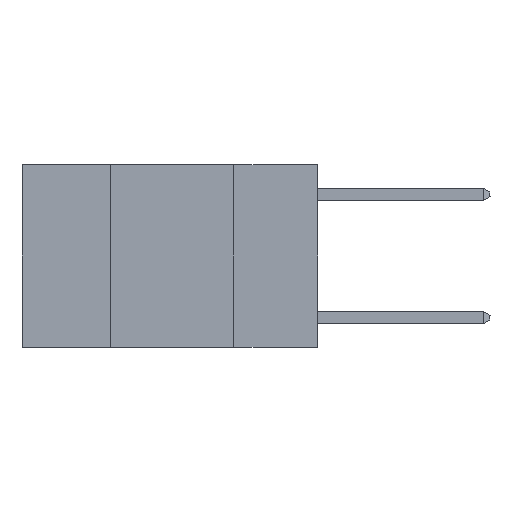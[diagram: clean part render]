
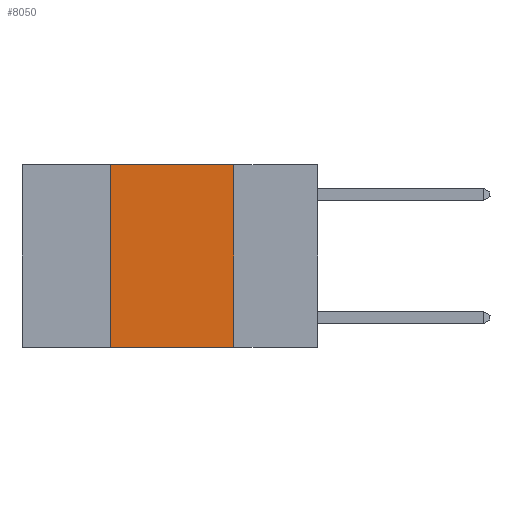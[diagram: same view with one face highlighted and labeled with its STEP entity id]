
A CAD part, left-side view. The second image highlights one B-rep face of the part: STEP entity #8050.
In plain terms, the highlighted planar face has unit normal (-1, 0, 0).
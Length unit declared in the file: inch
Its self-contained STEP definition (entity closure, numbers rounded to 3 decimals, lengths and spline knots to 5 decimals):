
#43 = AXIS2_PLACEMENT_3D ( 'NONE', #1854, #23886, #24026 ) ;
#94 = VECTOR ( 'NONE', #15990, 39.37008 ) ;
#1108 = EDGE_CURVE ( 'NONE', #13047, #16298, #21081, .T. ) ;
#1854 = CARTESIAN_POINT ( 'NONE',  ( 0., 0.6, 0. ) ) ;
#1896 = ORIENTED_EDGE ( 'NONE', *, *, #28391, .F. ) ;
#2667 = LINE ( 'NONE', #18173, #94 ) ;
#3849 = EDGE_CURVE ( 'NONE', #11766, #23685, #21653, .T. ) ;
#4004 = CARTESIAN_POINT ( 'NONE',  ( 0., 0.17, 0. ) ) ;
#4417 = VECTOR ( 'NONE', #8934, 39.37008 ) ;
#6445 = CARTESIAN_POINT ( 'NONE',  ( 0., 0.17, -0.37 ) ) ;
#7038 = VECTOR ( 'NONE', #18765, 39.37008 ) ;
#7938 = CARTESIAN_POINT ( 'NONE',  ( 0., 0.42, 0. ) ) ;
#8050 = ADVANCED_FACE ( 'NONE', ( #15036 ), #17356, .F. ) ;
#8934 = DIRECTION ( 'NONE',  ( 0., -1., 0. ) ) ;
#8973 = ORIENTED_EDGE ( 'NONE', *, *, #3849, .F. ) ;
#10432 = ORIENTED_EDGE ( 'NONE', *, *, #25284, .T. ) ;
#11766 = VERTEX_POINT ( 'NONE', #24717 ) ;
#13047 = VERTEX_POINT ( 'NONE', #16086 ) ;
#14161 = CARTESIAN_POINT ( 'NONE',  ( 0., 0.42, 0. ) ) ;
#15036 = FACE_OUTER_BOUND ( 'NONE', #17390, .T. ) ;
#15990 = DIRECTION ( 'NONE',  ( 0., -1., 0. ) ) ;
#16086 = CARTESIAN_POINT ( 'NONE',  ( 0., 0.42, -0.37 ) ) ;
#16298 = VERTEX_POINT ( 'NONE', #14161 ) ;
#16890 = LINE ( 'NONE', #26885, #4417 ) ;
#17356 = PLANE ( 'NONE',  #43 ) ;
#17390 = EDGE_LOOP ( 'NONE', ( #8973, #1896, #19580, #10432 ) ) ;
#18173 = CARTESIAN_POINT ( 'NONE',  ( 0., 0.6, -0.37 ) ) ;
#18765 = DIRECTION ( 'NONE',  ( 0., 0., 1. ) ) ;
#18779 = VECTOR ( 'NONE', #26297, 39.37008 ) ;
#19580 = ORIENTED_EDGE ( 'NONE', *, *, #1108, .F. ) ;
#21081 = LINE ( 'NONE', #7938, #7038 ) ;
#21653 = LINE ( 'NONE', #4004, #18779 ) ;
#23685 = VERTEX_POINT ( 'NONE', #6445 ) ;
#23886 = DIRECTION ( 'NONE',  ( 1., 0., 0. ) ) ;
#24026 = DIRECTION ( 'NONE',  ( 0., 0., -1. ) ) ;
#24717 = CARTESIAN_POINT ( 'NONE',  ( 0., 0.17, 0. ) ) ;
#25284 = EDGE_CURVE ( 'NONE', #13047, #23685, #2667, .T. ) ;
#26297 = DIRECTION ( 'NONE',  ( 0., 0., -1. ) ) ;
#26885 = CARTESIAN_POINT ( 'NONE',  ( 0., 0.6, 0. ) ) ;
#28391 = EDGE_CURVE ( 'NONE', #16298, #11766, #16890, .T. ) ;
